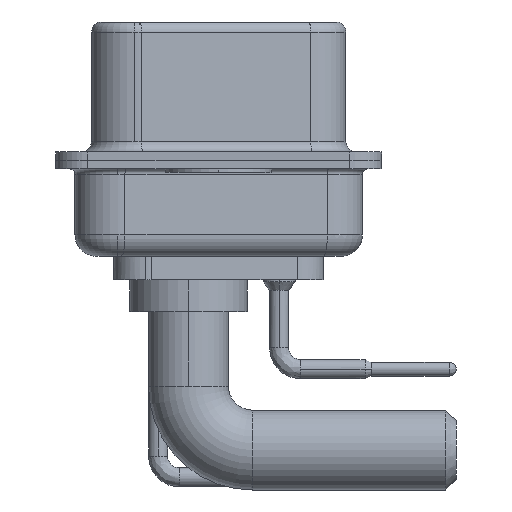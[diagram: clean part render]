
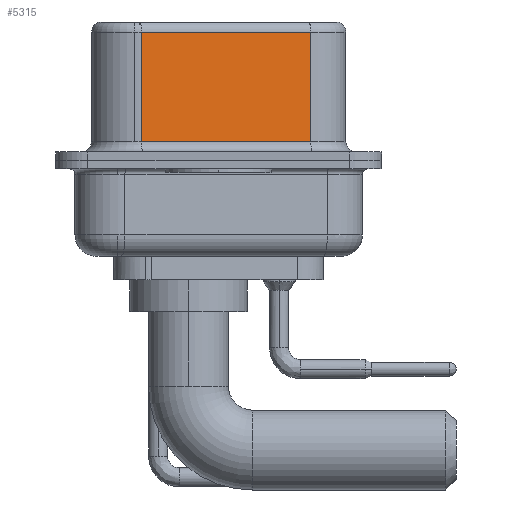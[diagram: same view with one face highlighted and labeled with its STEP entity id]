
A CAD part, left-side view. The second image highlights one B-rep face of the part: STEP entity #5315.
In plain terms, the highlighted planar face has unit normal (-0.985, -0.174, 0).
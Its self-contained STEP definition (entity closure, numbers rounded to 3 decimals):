
#4171 = DIRECTION ( 'NONE',  ( 0.985, 0.174, 0. ) ) ;
#5315 = ADVANCED_FACE ( 'NONE', ( #29439 ), #11880, .F. ) ;
#6113 = ORIENTED_EDGE ( 'NONE', *, *, #31602, .T. ) ;
#6209 = CARTESIAN_POINT ( 'NONE',  ( 3.73, 3.628, 6.02 ) ) ;
#6584 = CARTESIAN_POINT ( 'NONE',  ( 5.132, -4.322, 0.9 ) ) ;
#7414 = LINE ( 'NONE', #17413, #23012 ) ;
#9306 = VERTEX_POINT ( 'NONE', #6209 ) ;
#9360 = VECTOR ( 'NONE', #31824, 1000. ) ;
#10249 = VERTEX_POINT ( 'NONE', #14159 ) ;
#11302 = DIRECTION ( 'NONE',  ( 0., 0., -1. ) ) ;
#11803 = EDGE_CURVE ( 'NONE', #19362, #10249, #14116, .T. ) ;
#11880 = PLANE ( 'NONE',  #13622 ) ;
#12611 = CARTESIAN_POINT ( 'NONE',  ( 3.73, 3.628, 0.9 ) ) ;
#13622 = AXIS2_PLACEMENT_3D ( 'NONE', #14500, #4171, #18927 ) ;
#14116 = LINE ( 'NONE', #6584, #9360 ) ;
#14159 = CARTESIAN_POINT ( 'NONE',  ( 5.132, -4.322, 0.9 ) ) ;
#14500 = CARTESIAN_POINT ( 'NONE',  ( 5.132, -4.322, 6.52 ) ) ;
#15353 = EDGE_CURVE ( 'NONE', #28669, #10249, #7414, .T. ) ;
#17111 = VECTOR ( 'NONE', #19503, 1000. ) ;
#17413 = CARTESIAN_POINT ( 'NONE',  ( 5.132, -4.322, 6.52 ) ) ;
#18526 = EDGE_CURVE ( 'NONE', #28669, #9306, #21312, .T. ) ;
#18927 = DIRECTION ( 'NONE',  ( -0.174, 0.985, 0. ) ) ;
#19356 = LINE ( 'NONE', #24750, #26814 ) ;
#19362 = VERTEX_POINT ( 'NONE', #12611 ) ;
#19503 = DIRECTION ( 'NONE',  ( -0.174, 0.985, 0. ) ) ;
#19829 = DIRECTION ( 'NONE',  ( 0., 0., -1. ) ) ;
#19912 = ORIENTED_EDGE ( 'NONE', *, *, #18526, .T. ) ;
#20915 = ORIENTED_EDGE ( 'NONE', *, *, #11803, .T. ) ;
#21312 = LINE ( 'NONE', #26880, #17111 ) ;
#22976 = EDGE_LOOP ( 'NONE', ( #29709, #19912, #6113, #20915 ) ) ;
#23012 = VECTOR ( 'NONE', #11302, 1000. ) ;
#24750 = CARTESIAN_POINT ( 'NONE',  ( 3.73, 3.628, 6.52 ) ) ;
#26814 = VECTOR ( 'NONE', #19829, 1000. ) ;
#26880 = CARTESIAN_POINT ( 'NONE',  ( 5.132, -4.322, 6.02 ) ) ;
#28669 = VERTEX_POINT ( 'NONE', #29127 ) ;
#29127 = CARTESIAN_POINT ( 'NONE',  ( 5.132, -4.322, 6.02 ) ) ;
#29439 = FACE_OUTER_BOUND ( 'NONE', #22976, .T. ) ;
#29709 = ORIENTED_EDGE ( 'NONE', *, *, #15353, .F. ) ;
#31602 = EDGE_CURVE ( 'NONE', #9306, #19362, #19356, .T. ) ;
#31824 = DIRECTION ( 'NONE',  ( 0.174, -0.985, 0. ) ) ;
